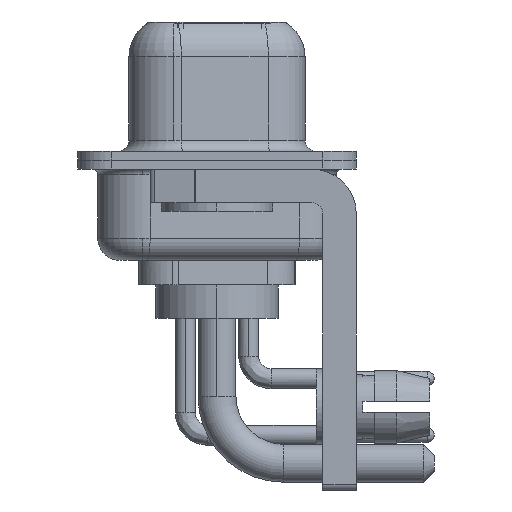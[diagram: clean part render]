
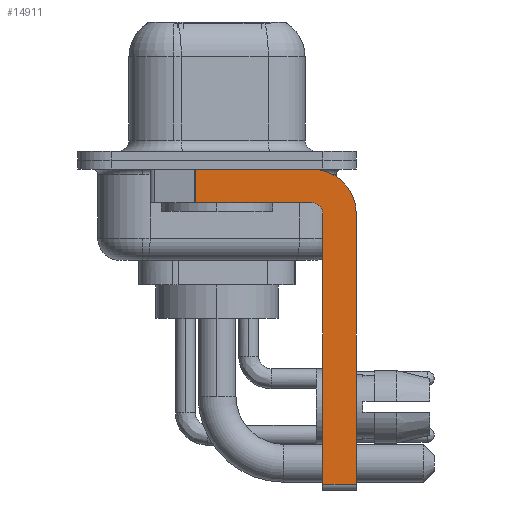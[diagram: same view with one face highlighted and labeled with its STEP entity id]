
A CAD part, left-side view. The second image highlights one B-rep face of the part: STEP entity #14911.
In plain terms, the highlighted planar face has unit normal (-1, 0, 0).
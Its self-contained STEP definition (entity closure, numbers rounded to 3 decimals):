
#857 = ORIENTED_EDGE ( 'NONE', *, *, #6339, .F. ) ;
#1012 = CARTESIAN_POINT ( 'NONE',  ( -2.9, -6.25, -14.55 ) ) ;
#1132 = VERTEX_POINT ( 'NONE', #7427 ) ;
#1401 = VECTOR ( 'NONE', #15876, 1000. ) ;
#1795 = CARTESIAN_POINT ( 'NONE',  ( -2.9, 0.978, -1.9 ) ) ;
#2184 = CARTESIAN_POINT ( 'NONE',  ( -2.9, -6.25, -2.4 ) ) ;
#2256 = VERTEX_POINT ( 'NONE', #8569 ) ;
#2516 = EDGE_CURVE ( 'NONE', #18410, #2256, #22315, .T. ) ;
#2551 = ORIENTED_EDGE ( 'NONE', *, *, #6422, .F. ) ;
#2702 = CARTESIAN_POINT ( 'NONE',  ( -2.9, 0.978, -0.4 ) ) ;
#3151 = VECTOR ( 'NONE', #18248, 1000. ) ;
#3464 = CARTESIAN_POINT ( 'NONE',  ( -2.9, -4.75, -2.4 ) ) ;
#3596 = AXIS2_PLACEMENT_3D ( 'NONE', #22347, #5416, #20382 ) ;
#4347 = EDGE_CURVE ( 'NONE', #24324, #7219, #8828, .T. ) ;
#4369 = ORIENTED_EDGE ( 'NONE', *, *, #16336, .T. ) ;
#4647 = DIRECTION ( 'NONE',  ( 0., 0., -1. ) ) ;
#5235 = VERTEX_POINT ( 'NONE', #13996 ) ;
#5416 = DIRECTION ( 'NONE',  ( -1., 0., 0. ) ) ;
#6339 = EDGE_CURVE ( 'NONE', #18410, #1132, #15905, .T. ) ;
#6422 = EDGE_CURVE ( 'NONE', #7219, #5235, #22551, .T. ) ;
#7107 = ORIENTED_EDGE ( 'NONE', *, *, #18414, .F. ) ;
#7171 = ORIENTED_EDGE ( 'NONE', *, *, #23308, .F. ) ;
#7219 = VERTEX_POINT ( 'NONE', #3464 ) ;
#7257 = CARTESIAN_POINT ( 'NONE',  ( -2.9, -4.75, -14.55 ) ) ;
#7427 = CARTESIAN_POINT ( 'NONE',  ( -2.9, -4.25, -0.4 ) ) ;
#7785 = EDGE_LOOP ( 'NONE', ( #857, #13026, #7171, #2551, #22177, #4369, #7107, #13954 ) ) ;
#8008 = AXIS2_PLACEMENT_3D ( 'NONE', #18590, #22663, #20806 ) ;
#8131 = DIRECTION ( 'NONE',  ( 0., -1., 0. ) ) ;
#8569 = CARTESIAN_POINT ( 'NONE',  ( -2.9, 0.978, -1.9 ) ) ;
#8828 = LINE ( 'NONE', #23793, #1401 ) ;
#8830 = DIRECTION ( 'NONE',  ( 0., 0., -1. ) ) ;
#9720 = LINE ( 'NONE', #2184, #12461 ) ;
#10399 = VECTOR ( 'NONE', #11039, 1000. ) ;
#11039 = DIRECTION ( 'NONE',  ( 0., -1., 0. ) ) ;
#11785 = CARTESIAN_POINT ( 'NONE',  ( -2.9, -4.25, -1.9 ) ) ;
#12461 = VECTOR ( 'NONE', #4647, 1000. ) ;
#12982 = DIRECTION ( 'NONE',  ( 1., 0., 0. ) ) ;
#13009 = CARTESIAN_POINT ( 'NONE',  ( -2.9, -4.25, -14.55 ) ) ;
#13026 = ORIENTED_EDGE ( 'NONE', *, *, #2516, .T. ) ;
#13068 = EDGE_CURVE ( 'NONE', #1132, #20174, #21507, .T. ) ;
#13509 = CARTESIAN_POINT ( 'NONE',  ( -2.9, -6.25, -2.4 ) ) ;
#13954 = ORIENTED_EDGE ( 'NONE', *, *, #13068, .F. ) ;
#13996 = CARTESIAN_POINT ( 'NONE',  ( -2.9, -4.25, -1.9 ) ) ;
#14911 = ADVANCED_FACE ( 'NONE', ( #20690 ), #16957, .F. ) ;
#15876 = DIRECTION ( 'NONE',  ( 0., 0., 1. ) ) ;
#15905 = LINE ( 'NONE', #23444, #23315 ) ;
#16336 = EDGE_CURVE ( 'NONE', #24324, #17876, #18595, .T. ) ;
#16782 = AXIS2_PLACEMENT_3D ( 'NONE', #19063, #12982, #21030 ) ;
#16957 = PLANE ( 'NONE',  #8008 ) ;
#17876 = VERTEX_POINT ( 'NONE', #1012 ) ;
#18205 = VECTOR ( 'NONE', #8830, 1000. ) ;
#18248 = DIRECTION ( 'NONE',  ( 0., 1., 0. ) ) ;
#18410 = VERTEX_POINT ( 'NONE', #2702 ) ;
#18414 = EDGE_CURVE ( 'NONE', #20174, #17876, #9720, .T. ) ;
#18590 = CARTESIAN_POINT ( 'NONE',  ( -2.9, -4.25, -2.4 ) ) ;
#18595 = LINE ( 'NONE', #13009, #10399 ) ;
#19063 = CARTESIAN_POINT ( 'NONE',  ( -2.9, -4.25, -2.4 ) ) ;
#20174 = VERTEX_POINT ( 'NONE', #13509 ) ;
#20382 = DIRECTION ( 'NONE',  ( 0., 0., 1. ) ) ;
#20690 = FACE_OUTER_BOUND ( 'NONE', #7785, .T. ) ;
#20806 = DIRECTION ( 'NONE',  ( 0., 0., -1. ) ) ;
#21030 = DIRECTION ( 'NONE',  ( 0., 0., -1. ) ) ;
#21087 = LINE ( 'NONE', #11785, #3151 ) ;
#21507 = CIRCLE ( 'NONE', #16782, 2. ) ;
#22177 = ORIENTED_EDGE ( 'NONE', *, *, #4347, .F. ) ;
#22315 = LINE ( 'NONE', #1795, #18205 ) ;
#22347 = CARTESIAN_POINT ( 'NONE',  ( -2.9, -4.25, -2.4 ) ) ;
#22551 = CIRCLE ( 'NONE', #3596, 0.5 ) ;
#22663 = DIRECTION ( 'NONE',  ( 1., 0., 0. ) ) ;
#23308 = EDGE_CURVE ( 'NONE', #5235, #2256, #21087, .T. ) ;
#23315 = VECTOR ( 'NONE', #8131, 1000. ) ;
#23444 = CARTESIAN_POINT ( 'NONE',  ( -2.9, 3., -0.4 ) ) ;
#23793 = CARTESIAN_POINT ( 'NONE',  ( -2.9, -4.75, -14.8 ) ) ;
#24324 = VERTEX_POINT ( 'NONE', #7257 ) ;
